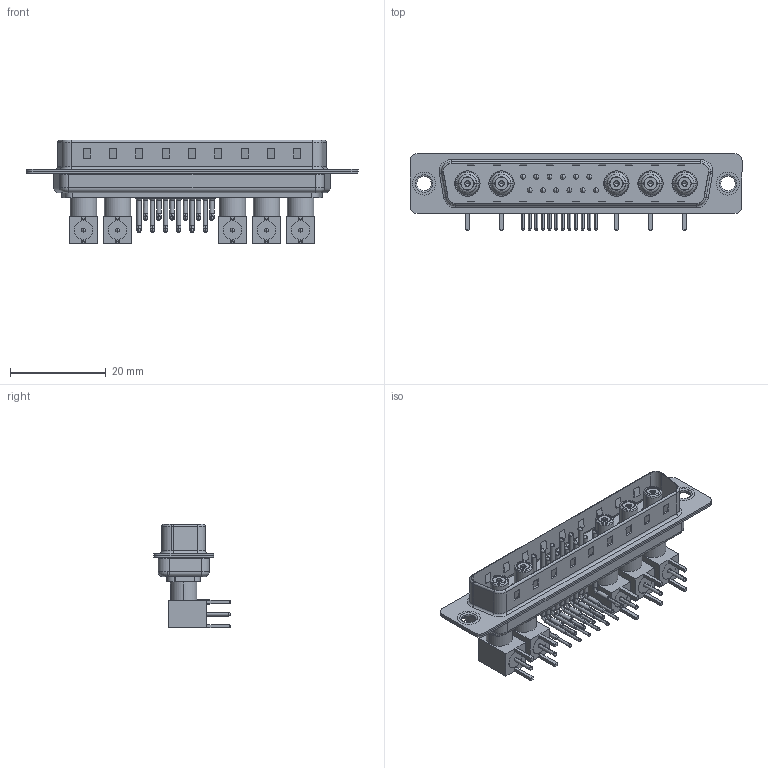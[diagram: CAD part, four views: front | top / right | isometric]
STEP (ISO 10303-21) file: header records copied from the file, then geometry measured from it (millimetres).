
FILE_DESCRIPTION (( 'STEP AP203' ), '1' );
FILE_NAME ('629-17W5640-7N1.STEP', '2022-05-16T00:39:12', ( '' ), ( '' ), 'SwSTEP 2.0', 'SolidWorks 2020', '' );
FILE_SCHEMA (( 'CONFIG_CONTROL_DESIGN' ));
Length unit declared in the file: millimetre
Products named in the file (19): Co-Ax Jack Assy_RA; Co-Ax Jack_RA PC Tail; 629Combo Contact Row 2; Insulator Socket; 629Combo Housing_17W5; 629Combo Contact Row 1; Insulator RA Pin; Locking Collar; Insulator Socket 2; RA Back Shell; 629Combo Shell Front_37 Contacts; 629-17W5640-7N1; 629Combo Thru Hole Rivet; 629Combo Shell Rear_37 Contacts; Socket_RA
Assembly tree (57 placements, depth 3):
  629-17W5640-7N1
    629Combo Housing_17W5
    629Combo Shell Rear_37 Contacts
    629Combo Shell Front_37 Contacts
    629Combo Thru Hole Rivet  x2
    Co-Ax Jack Assy_RA
      Co-Ax Jack_RA PC Tail
      Insulator Socket
      Insulator Socket 2
      Locking Collar
      Socket_RA
      RA Back Shell
      Insulator RA Pin
    Co-Ax Jack Assy_RA
      Co-Ax Jack_RA PC Tail
      Insulator Socket
      Insulator Socket 2
      Locking Collar
      Socket_RA
      RA Back Shell
      Insulator RA Pin
    Co-Ax Jack Assy_RA
      Co-Ax Jack_RA PC Tail
      Insulator Socket
      Insulator Socket 2
      Locking Collar
      Socket_RA
      RA Back Shell
      Insulator RA Pin
    Co-Ax Jack Assy_RA
      Co-Ax Jack_RA PC Tail
      Insulator Socket
      Insulator Socket 2
      Locking Collar
      Socket_RA
      RA Back Shell
      Insulator RA Pin
    Co-Ax Jack Assy_RA
      Co-Ax Jack_RA PC Tail
      Insulator Socket
      Insulator Socket 2
      Locking Collar
      Socket_RA
      RA Back Shell
      Insulator RA Pin
    629Combo Contact Row 1  x6
    629Combo Contact Row 2  x6
Bounding box: 69.4 x 16 x 21.71 mm (x, y, z)
Volume: 5213.8 mm3; surface area: 14065.7 mm2
Topology: 52 solids, 52 shells, 2466 faces, 6432 edges, 4111 vertices
Faces by surface type: plane 1256, cylinder 892, cone 143, torus 88, bspline 77, sphere 10
Entity records: 28968 total; most frequent: CARTESIAN_POINT 4807, DIRECTION 4645, ORIENTED_EDGE 4220, EDGE_CURVE 2110, AXIS2_PLACEMENT_3D 1678, VERTEX_POINT 1355, LINE 1289, VECTOR 1289
